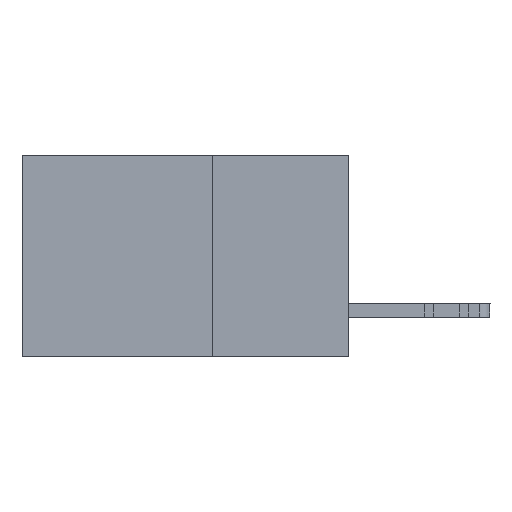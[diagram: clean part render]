
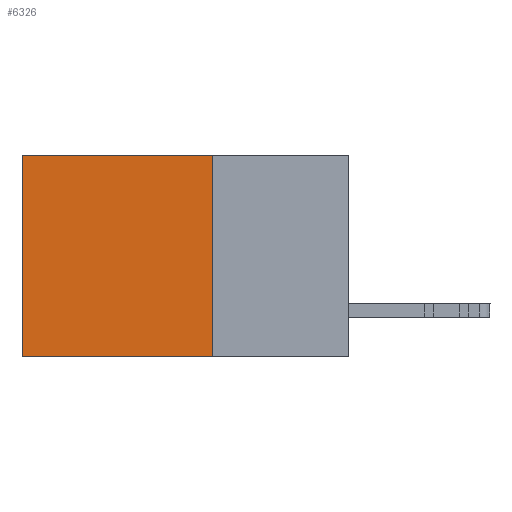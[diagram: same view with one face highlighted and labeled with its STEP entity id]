
A CAD part, left-side view. The second image highlights one B-rep face of the part: STEP entity #6326.
In plain terms, the highlighted planar face has unit normal (-1, 0, 0).
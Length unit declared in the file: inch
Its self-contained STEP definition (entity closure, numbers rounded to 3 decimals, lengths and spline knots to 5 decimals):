
#173 = CARTESIAN_POINT ( 'NONE',  ( 0.298, 0.25, 0. ) ) ;
#635 = LINE ( 'NONE', #11952, #3642 ) ;
#1107 = DIRECTION ( 'NONE',  ( 1., 0., 0. ) ) ;
#1337 = CARTESIAN_POINT ( 'NONE',  ( 0.298, 0.6, -0.37 ) ) ;
#1576 = FACE_OUTER_BOUND ( 'NONE', #2373, .T. ) ;
#2373 = EDGE_LOOP ( 'NONE', ( #19643, #15205, #30234, #30433 ) ) ;
#2558 = PLANE ( 'NONE',  #20829 ) ;
#3196 = EDGE_CURVE ( 'NONE', #6809, #11438, #635, .T. ) ;
#3334 = EDGE_CURVE ( 'NONE', #23794, #6809, #27757, .T. ) ;
#3642 = VECTOR ( 'NONE', #28769, 39.37008 ) ;
#5874 = DIRECTION ( 'NONE',  ( 0., 0., -1. ) ) ;
#6326 = ADVANCED_FACE ( 'NONE', ( #1576 ), #2558, .F. ) ;
#6568 = LINE ( 'NONE', #22595, #9907 ) ;
#6809 = VERTEX_POINT ( 'NONE', #13123 ) ;
#7188 = CARTESIAN_POINT ( 'NONE',  ( 0.298, 0.25, 0. ) ) ;
#7610 = EDGE_CURVE ( 'NONE', #23794, #10461, #30110, .T. ) ;
#9907 = VECTOR ( 'NONE', #5874, 39.37008 ) ;
#10461 = VERTEX_POINT ( 'NONE', #28906 ) ;
#11438 = VERTEX_POINT ( 'NONE', #1337 ) ;
#11952 = CARTESIAN_POINT ( 'NONE',  ( 0.298, 0.25, -0.37 ) ) ;
#12335 = CARTESIAN_POINT ( 'NONE',  ( 0.298, 0.25, 0. ) ) ;
#12366 = DIRECTION ( 'NONE',  ( 0., 0., -1. ) ) ;
#13123 = CARTESIAN_POINT ( 'NONE',  ( 0.298, 0.25, -0.37 ) ) ;
#15205 = ORIENTED_EDGE ( 'NONE', *, *, #3196, .F. ) ;
#15847 = EDGE_CURVE ( 'NONE', #10461, #11438, #6568, .T. ) ;
#19149 = DIRECTION ( 'NONE',  ( 0., 1., 0. ) ) ;
#19643 = ORIENTED_EDGE ( 'NONE', *, *, #15847, .T. ) ;
#20829 = AXIS2_PLACEMENT_3D ( 'NONE', #12335, #1107, #22527 ) ;
#22041 = CARTESIAN_POINT ( 'NONE',  ( 0.298, 0.25, 0. ) ) ;
#22527 = DIRECTION ( 'NONE',  ( 0., 0., -1. ) ) ;
#22595 = CARTESIAN_POINT ( 'NONE',  ( 0.298, 0.6, 0. ) ) ;
#23794 = VERTEX_POINT ( 'NONE', #173 ) ;
#26740 = VECTOR ( 'NONE', #19149, 39.37008 ) ;
#27757 = LINE ( 'NONE', #22041, #31096 ) ;
#28769 = DIRECTION ( 'NONE',  ( 0., 1., 0. ) ) ;
#28906 = CARTESIAN_POINT ( 'NONE',  ( 0.298, 0.6, 0. ) ) ;
#30110 = LINE ( 'NONE', #7188, #26740 ) ;
#30234 = ORIENTED_EDGE ( 'NONE', *, *, #3334, .F. ) ;
#30433 = ORIENTED_EDGE ( 'NONE', *, *, #7610, .T. ) ;
#31096 = VECTOR ( 'NONE', #12366, 39.37008 ) ;
